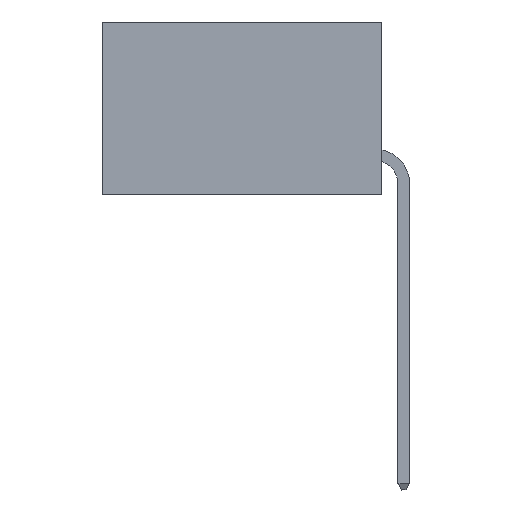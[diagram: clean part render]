
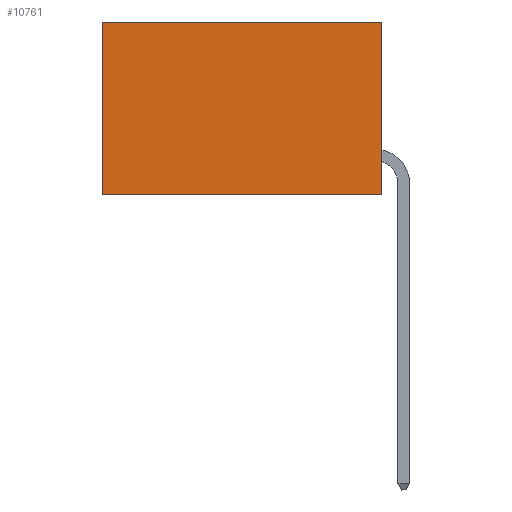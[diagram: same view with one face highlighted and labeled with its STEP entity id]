
A CAD part, left-side view. The second image highlights one B-rep face of the part: STEP entity #10761.
In plain terms, the highlighted planar face has unit normal (-1, 0, 0).
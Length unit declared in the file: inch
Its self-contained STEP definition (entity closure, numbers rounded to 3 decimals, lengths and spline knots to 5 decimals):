
#997 = ORIENTED_EDGE ( 'NONE', *, *, #35434, .T. ) ;
#2648 = VECTOR ( 'NONE', #6065, 39.37008 ) ;
#4037 = PLANE ( 'NONE',  #26147 ) ;
#5159 = VERTEX_POINT ( 'NONE', #32257 ) ;
#5234 = DIRECTION ( 'NONE',  ( 0., 1., 0. ) ) ;
#6065 = DIRECTION ( 'NONE',  ( 0., 1., 0. ) ) ;
#6382 = VECTOR ( 'NONE', #5234, 39.37008 ) ;
#6423 = CARTESIAN_POINT ( 'NONE',  ( 0.2875, 0.6, -0.37 ) ) ;
#7626 = LINE ( 'NONE', #8039, #2648 ) ;
#8039 = CARTESIAN_POINT ( 'NONE',  ( 0.2875, 0., -0.37 ) ) ;
#8667 = VERTEX_POINT ( 'NONE', #6423 ) ;
#8938 = EDGE_CURVE ( 'NONE', #10396, #8667, #7626, .T. ) ;
#10396 = VERTEX_POINT ( 'NONE', #39742 ) ;
#10761 = ADVANCED_FACE ( 'NONE', ( #27021 ), #4037, .F. ) ;
#12162 = LINE ( 'NONE', #32326, #15187 ) ;
#13381 = DIRECTION ( 'NONE',  ( 1., 0., 0. ) ) ;
#14219 = CARTESIAN_POINT ( 'NONE',  ( 0.2875, 0.6, 0. ) ) ;
#14768 = CARTESIAN_POINT ( 'NONE',  ( 0.2875, 0.6, 0. ) ) ;
#14910 = DIRECTION ( 'NONE',  ( 0., 0., -1. ) ) ;
#15187 = VECTOR ( 'NONE', #19709, 39.37008 ) ;
#17032 = DIRECTION ( 'NONE',  ( 0., 0., -1. ) ) ;
#18396 = VECTOR ( 'NONE', #14910, 39.37008 ) ;
#19709 = DIRECTION ( 'NONE',  ( 0., 0., -1. ) ) ;
#19743 = CARTESIAN_POINT ( 'NONE',  ( 0.2875, 0., 0. ) ) ;
#20701 = ORIENTED_EDGE ( 'NONE', *, *, #8938, .F. ) ;
#24501 = EDGE_LOOP ( 'NONE', ( #997, #20701, #36534, #37106 ) ) ;
#26147 = AXIS2_PLACEMENT_3D ( 'NONE', #19743, #13381, #17032 ) ;
#27021 = FACE_OUTER_BOUND ( 'NONE', #24501, .T. ) ;
#32257 = CARTESIAN_POINT ( 'NONE',  ( 0.2875, 0., 0. ) ) ;
#32326 = CARTESIAN_POINT ( 'NONE',  ( 0.2875, 0., 0. ) ) ;
#33931 = CARTESIAN_POINT ( 'NONE',  ( 0.2875, 0., 0. ) ) ;
#34213 = EDGE_CURVE ( 'NONE', #5159, #35370, #39743, .T. ) ;
#35370 = VERTEX_POINT ( 'NONE', #14219 ) ;
#35434 = EDGE_CURVE ( 'NONE', #35370, #8667, #40673, .T. ) ;
#36534 = ORIENTED_EDGE ( 'NONE', *, *, #37197, .F. ) ;
#37106 = ORIENTED_EDGE ( 'NONE', *, *, #34213, .T. ) ;
#37197 = EDGE_CURVE ( 'NONE', #5159, #10396, #12162, .T. ) ;
#39742 = CARTESIAN_POINT ( 'NONE',  ( 0.2875, 0., -0.37 ) ) ;
#39743 = LINE ( 'NONE', #33931, #6382 ) ;
#40673 = LINE ( 'NONE', #14768, #18396 ) ;
